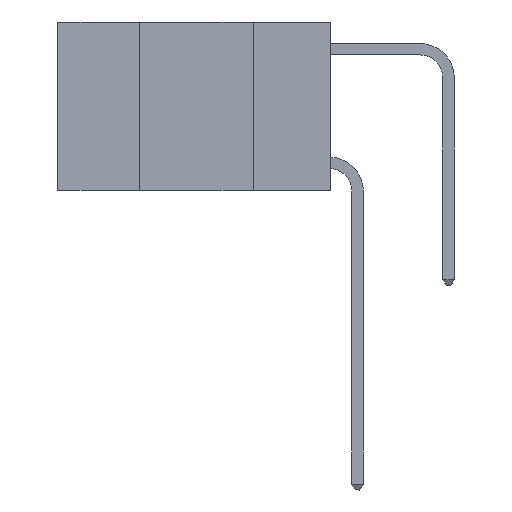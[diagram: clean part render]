
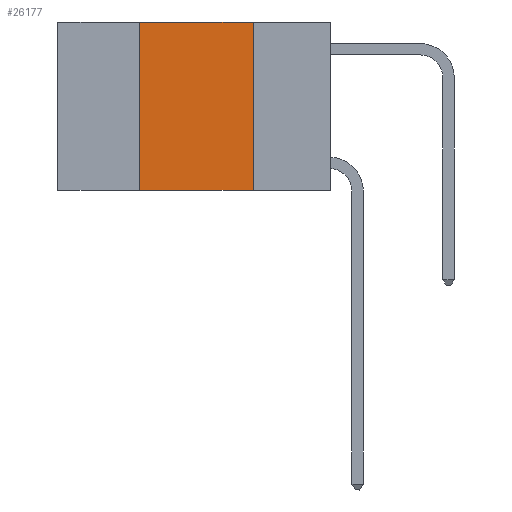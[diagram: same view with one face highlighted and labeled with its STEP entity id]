
A CAD part, left-side view. The second image highlights one B-rep face of the part: STEP entity #26177.
In plain terms, the highlighted planar face has unit normal (-1, 0, 0).
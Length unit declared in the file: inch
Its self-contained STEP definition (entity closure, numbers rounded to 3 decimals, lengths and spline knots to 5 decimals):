
#487 = EDGE_CURVE ( 'NONE', #20872, #14029, #22250, .T. ) ;
#1177 = CARTESIAN_POINT ( 'NONE',  ( 0., 0.42, 0. ) ) ;
#2757 = VECTOR ( 'NONE', #23842, 39.37008 ) ;
#3097 = ORIENTED_EDGE ( 'NONE', *, *, #18591, .T. ) ;
#4603 = VERTEX_POINT ( 'NONE', #25400 ) ;
#5064 = EDGE_CURVE ( 'NONE', #4603, #20872, #13370, .T. ) ;
#5104 = ORIENTED_EDGE ( 'NONE', *, *, #17297, .F. ) ;
#6121 = CARTESIAN_POINT ( 'NONE',  ( 0., 0.42, 0. ) ) ;
#7370 = DIRECTION ( 'NONE',  ( 1., 0., 0. ) ) ;
#8970 = AXIS2_PLACEMENT_3D ( 'NONE', #21224, #7370, #16925 ) ;
#9429 = ORIENTED_EDGE ( 'NONE', *, *, #487, .F. ) ;
#9582 = LINE ( 'NONE', #21968, #28224 ) ;
#11846 = PLANE ( 'NONE',  #8970 ) ;
#13210 = DIRECTION ( 'NONE',  ( 0., 0., 1. ) ) ;
#13370 = LINE ( 'NONE', #6121, #15147 ) ;
#14029 = VERTEX_POINT ( 'NONE', #25398 ) ;
#15147 = VECTOR ( 'NONE', #13210, 39.37008 ) ;
#16925 = DIRECTION ( 'NONE',  ( 0., 0., -1. ) ) ;
#16934 = CARTESIAN_POINT ( 'NONE',  ( 0., 0.6, 0. ) ) ;
#17297 = EDGE_CURVE ( 'NONE', #14029, #23978, #9582, .T. ) ;
#18346 = CARTESIAN_POINT ( 'NONE',  ( 0., 0.6, -0.37 ) ) ;
#18591 = EDGE_CURVE ( 'NONE', #4603, #23978, #30049, .T. ) ;
#20872 = VERTEX_POINT ( 'NONE', #1177 ) ;
#21079 = ORIENTED_EDGE ( 'NONE', *, *, #5064, .F. ) ;
#21224 = CARTESIAN_POINT ( 'NONE',  ( 0., 0.6, 0. ) ) ;
#21765 = CARTESIAN_POINT ( 'NONE',  ( 0., 0.17, -0.37 ) ) ;
#21968 = CARTESIAN_POINT ( 'NONE',  ( 0., 0.17, 0. ) ) ;
#22250 = LINE ( 'NONE', #16934, #2757 ) ;
#23716 = DIRECTION ( 'NONE',  ( 0., 0., -1. ) ) ;
#23842 = DIRECTION ( 'NONE',  ( 0., -1., 0. ) ) ;
#23978 = VERTEX_POINT ( 'NONE', #21765 ) ;
#25398 = CARTESIAN_POINT ( 'NONE',  ( 0., 0.17, 0. ) ) ;
#25400 = CARTESIAN_POINT ( 'NONE',  ( 0., 0.42, -0.37 ) ) ;
#25784 = EDGE_LOOP ( 'NONE', ( #5104, #9429, #21079, #3097 ) ) ;
#25995 = FACE_OUTER_BOUND ( 'NONE', #25784, .T. ) ;
#26177 = ADVANCED_FACE ( 'NONE', ( #25995 ), #11846, .F. ) ;
#27736 = DIRECTION ( 'NONE',  ( 0., -1., 0. ) ) ;
#28224 = VECTOR ( 'NONE', #23716, 39.37008 ) ;
#30049 = LINE ( 'NONE', #18346, #30240 ) ;
#30240 = VECTOR ( 'NONE', #27736, 39.37008 ) ;
